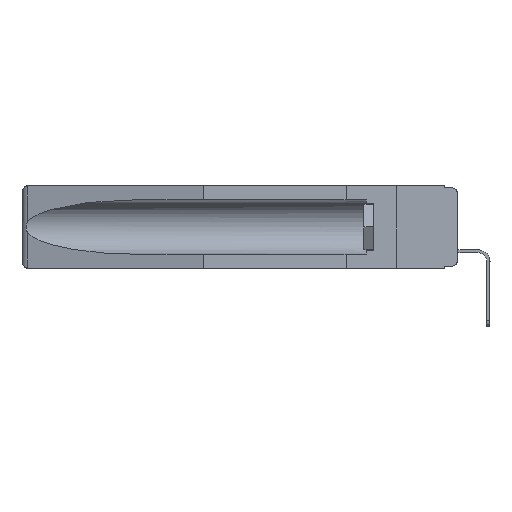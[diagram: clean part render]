
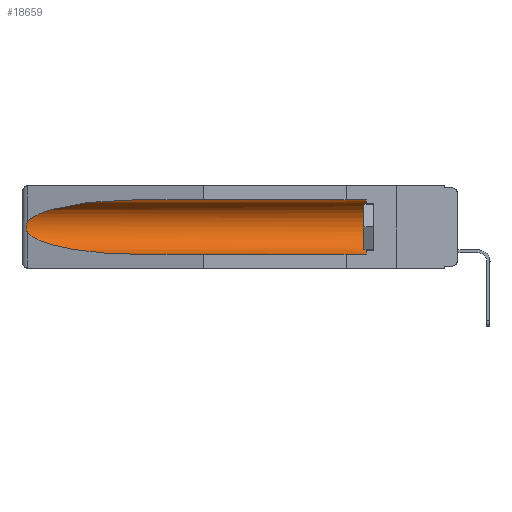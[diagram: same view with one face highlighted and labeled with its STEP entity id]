
A CAD part, left-side view. The second image highlights one B-rep face of the part: STEP entity #18659.
In plain terms, the highlighted cylindrical face has radius 2.857 mm (diameter 5.715 mm), a partial arc.
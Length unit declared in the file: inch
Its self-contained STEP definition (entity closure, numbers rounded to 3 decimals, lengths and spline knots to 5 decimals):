
#101 = EDGE_CURVE ( 'NONE', #479, #15373, #7127, .T. ) ;
#479 = VERTEX_POINT ( 'NONE', #15759 ) ;
#594 = CARTESIAN_POINT ( 'NONE',  ( 0.26537, 1.52718, -0.14972 ) ) ;
#600 = EDGE_CURVE ( 'NONE', #14240, #15373, #11599, .T. ) ;
#655 = CARTESIAN_POINT ( 'NONE',  ( 0.25451, 1.48313, -0.09465 ) ) ;
#842 = CARTESIAN_POINT ( 'NONE',  ( 0.26654, 1.53092, -0.15636 ) ) ;
#914 = DIRECTION ( 'NONE',  ( 0., 1., 0. ) ) ;
#982 = CARTESIAN_POINT ( 'NONE',  ( 0.2673, 1.5327, -0.16383 ) ) ;
#1324 = ORIENTED_EDGE ( 'NONE', *, *, #3136, .T. ) ;
#1756 = ORIENTED_EDGE ( 'NONE', *, *, #600, .F. ) ;
#1986 = DIRECTION ( 'NONE',  ( 0., 1., 0. ) ) ;
#2276 = VECTOR ( 'NONE', #14342, 39.37008 ) ;
#2469 = DIRECTION ( 'NONE',  ( 0., 0., 1. ) ) ;
#2522 = CARTESIAN_POINT ( 'NONE',  ( 0.2675, 1.53308, -0.17534 ) ) ;
#3136 = EDGE_CURVE ( 'NONE', #17650, #479, #11422, .T. ) ;
#3450 = CARTESIAN_POINT ( 'NONE',  ( 0.155, 1.07973, -0.059 ) ) ;
#4499 = CARTESIAN_POINT ( 'NONE',  ( 0.26537, 1.52718, -0.19328 ) ) ;
#5535 = CARTESIAN_POINT ( 'NONE',  ( 0.2675, 1.53308, -0.16763 ) ) ;
#5607 = CARTESIAN_POINT ( 'NONE',  ( 0.26537, 1.52718, -0.19328 ) ) ;
#5897 = ORIENTED_EDGE ( 'NONE', *, *, #16505, .T. ) ;
#6574 = CARTESIAN_POINT ( 'NONE',  ( 0.155, 1.07973, -0.059 ) ) ;
#7104 = CARTESIAN_POINT ( 'NONE',  ( 0.26655, 1.53094, -0.18657 ) ) ;
#7127 =( BOUNDED_CURVE ( )  B_SPLINE_CURVE ( 3, ( #4499, #13766, #12431, #9206 ),
 .UNSPECIFIED., .F., .F. ) 
 B_SPLINE_CURVE_WITH_KNOTS ( ( 4, 4 ),
 ( 0.1948, 1.5708 ),
 .UNSPECIFIED. ) 
 CURVE ( )  GEOMETRIC_REPRESENTATION_ITEM ( )  RATIONAL_B_SPLINE_CURVE ( ( 1., 0.848, 0.848, 1. ) ) 
 REPRESENTATION_ITEM ( '' )  );
#7217 = FACE_OUTER_BOUND ( 'NONE', #11017, .T. ) ;
#7506 = DIRECTION ( 'NONE',  ( 0., -1., 0. ) ) ;
#7792 = CARTESIAN_POINT ( 'NONE',  ( 0.155, 0.126, -0.059 ) ) ;
#8325 = VECTOR ( 'NONE', #1986, 39.37008 ) ;
#8498 = VERTEX_POINT ( 'NONE', #3450 ) ;
#8690 = CARTESIAN_POINT ( 'NONE',  ( 0.26597, 1.52961, -0.15275 ) ) ;
#9005 = AXIS2_PLACEMENT_3D ( 'NONE', #19667, #914, #2469 ) ;
#9206 = CARTESIAN_POINT ( 'NONE',  ( 0.155, 1.07973, -0.284 ) ) ;
#9762 = CIRCLE ( 'NONE', #19570, 0.1125 ) ;
#10030 = CARTESIAN_POINT ( 'NONE',  ( 0.21114, 1.30732, -0.059 ) ) ;
#10781 = LINE ( 'NONE', #17329, #8325 ) ;
#11017 = EDGE_LOOP ( 'NONE', ( #19939, #1324, #19266, #1756, #16782, #5897 ) ) ;
#11422 = B_SPLINE_CURVE_WITH_KNOTS ( 'NONE', 3,
 ( #14894, #8690, #842, #982, #5535, #2522, #16450, #7104, #19604, #5607 ),
 .UNSPECIFIED., .F., .F.,
 ( 4, 2, 2, 2, 4 ),
 ( 0., 0.00029, 0.00058, 0.00087, 0.00117 ),
 .UNSPECIFIED. ) ;
#11599 = LINE ( 'NONE', #17339, #2276 ) ;
#11618 = CARTESIAN_POINT ( 'NONE',  ( 0.155, 1.07973, -0.284 ) ) ;
#11621 = EDGE_CURVE ( 'NONE', #8498, #17650, #14389, .T. ) ;
#12098 = VERTEX_POINT ( 'NONE', #7792 ) ;
#12408 = CYLINDRICAL_SURFACE ( 'NONE', #9005, 0.1125 ) ;
#12431 = CARTESIAN_POINT ( 'NONE',  ( 0.21114, 1.30732, -0.284 ) ) ;
#12570 = CARTESIAN_POINT ( 'NONE',  ( 0.26537, 1.52718, -0.14972 ) ) ;
#13766 = CARTESIAN_POINT ( 'NONE',  ( 0.25451, 1.48313, -0.24835 ) ) ;
#14240 = VERTEX_POINT ( 'NONE', #16652 ) ;
#14342 = DIRECTION ( 'NONE',  ( 0., 1., 0. ) ) ;
#14389 =( BOUNDED_CURVE ( )  B_SPLINE_CURVE ( 3, ( #6574, #10030, #655, #594 ),
 .UNSPECIFIED., .F., .F. ) 
 B_SPLINE_CURVE_WITH_KNOTS ( ( 4, 4 ),
 ( 4.71239, 6.08839 ),
 .UNSPECIFIED. ) 
 CURVE ( )  GEOMETRIC_REPRESENTATION_ITEM ( )  RATIONAL_B_SPLINE_CURVE ( ( 1., 0.848, 0.848, 1. ) ) 
 REPRESENTATION_ITEM ( '' )  );
#14894 = CARTESIAN_POINT ( 'NONE',  ( 0.26537, 1.52718, -0.14972 ) ) ;
#15373 = VERTEX_POINT ( 'NONE', #11618 ) ;
#15759 = CARTESIAN_POINT ( 'NONE',  ( 0.26537, 1.52718, -0.19328 ) ) ;
#16450 = CARTESIAN_POINT ( 'NONE',  ( 0.2673, 1.53269, -0.17917 ) ) ;
#16505 = EDGE_CURVE ( 'NONE', #12098, #8498, #10781, .T. ) ;
#16652 = CARTESIAN_POINT ( 'NONE',  ( 0.155, 0.126, -0.284 ) ) ;
#16782 = ORIENTED_EDGE ( 'NONE', *, *, #17130, .T. ) ;
#17047 = CARTESIAN_POINT ( 'NONE',  ( 0.155, 0.126, -0.1715 ) ) ;
#17130 = EDGE_CURVE ( 'NONE', #14240, #12098, #9762, .T. ) ;
#17329 = CARTESIAN_POINT ( 'NONE',  ( 0.155, -0.30754, -0.059 ) ) ;
#17339 = CARTESIAN_POINT ( 'NONE',  ( 0.155, -0.30754, -0.284 ) ) ;
#17650 = VERTEX_POINT ( 'NONE', #12570 ) ;
#18426 = DIRECTION ( 'NONE',  ( 0., 0., 1. ) ) ;
#18659 = ADVANCED_FACE ( 'NONE', ( #7217 ), #12408, .F. ) ;
#19266 = ORIENTED_EDGE ( 'NONE', *, *, #101, .T. ) ;
#19570 = AXIS2_PLACEMENT_3D ( 'NONE', #17047, #7506, #18426 ) ;
#19604 = CARTESIAN_POINT ( 'NONE',  ( 0.26597, 1.5296, -0.19026 ) ) ;
#19667 = CARTESIAN_POINT ( 'NONE',  ( 0.155, -0.30754, -0.1715 ) ) ;
#19939 = ORIENTED_EDGE ( 'NONE', *, *, #11621, .T. ) ;
